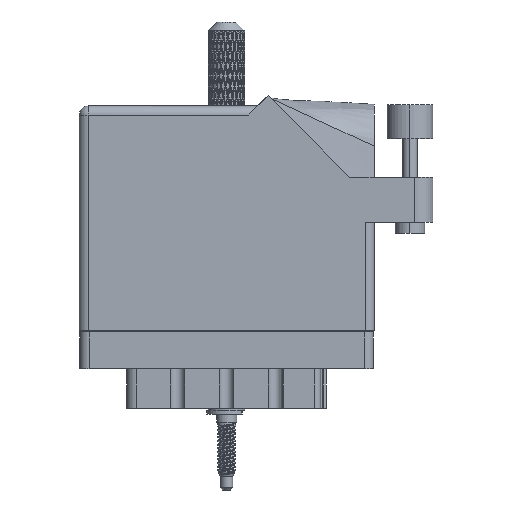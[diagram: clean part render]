
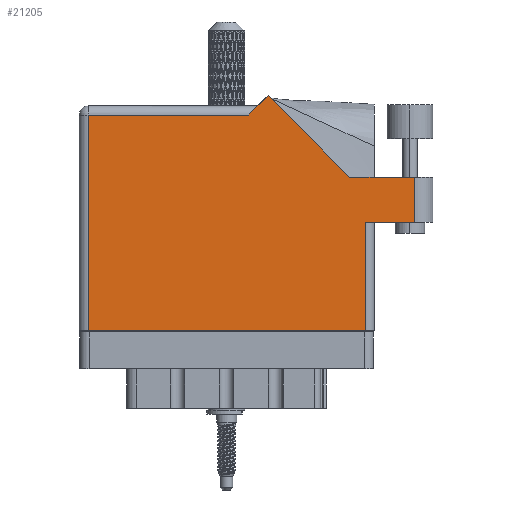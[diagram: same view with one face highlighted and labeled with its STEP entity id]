
A CAD part, front view. The second image highlights one B-rep face of the part: STEP entity #21205.
In plain terms, the highlighted face is planar.
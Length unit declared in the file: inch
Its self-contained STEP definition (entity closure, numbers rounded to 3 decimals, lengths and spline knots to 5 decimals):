
#4495 = LINE ( 'NONE', #63490, #35929 ) ;
#10375 = VERTEX_POINT ( 'NONE', #66895 ) ;
#10689 = CARTESIAN_POINT ( 'NONE',  ( 1.948, 0.737, 0. ) ) ;
#11623 = DIRECTION ( 'NONE',  ( 1., 0., 0. ) ) ;
#13002 = DIRECTION ( 'NONE',  ( 0., 1., 0. ) ) ;
#14336 = ORIENTED_EDGE ( 'NONE', *, *, #63837, .T. ) ;
#14407 = EDGE_CURVE ( 'NONE', #24327, #50296, #42086, .T. ) ;
#15687 = LINE ( 'NONE', #63874, #23790 ) ;
#17884 = CARTESIAN_POINT ( 'NONE',  ( 0.062, 1.468, 0. ) ) ;
#19351 = VERTEX_POINT ( 'NONE', #10689 ) ;
#20363 = DIRECTION ( 'NONE',  ( 0., 0., -1. ) ) ;
#20901 = DIRECTION ( 'NONE',  ( 1., 0., 0. ) ) ;
#21122 = VECTOR ( 'NONE', #20901, 39.37008 ) ;
#21205 = ADVANCED_FACE ( 'NONE', ( #87425 ), #86884, .F. ) ;
#21917 = VECTOR ( 'NONE', #93456, 39.37008 ) ;
#23449 = LINE ( 'NONE', #47319, #48902 ) ;
#23790 = VECTOR ( 'NONE', #65472, 39.37008 ) ;
#24327 = VERTEX_POINT ( 'NONE', #24471 ) ;
#24471 = CARTESIAN_POINT ( 'NONE',  ( 1.28771, 1.60071, 0. ) ) ;
#26936 = CARTESIAN_POINT ( 'NONE',  ( 1.217, 1.53, 0. ) ) ;
#27651 = ORIENTED_EDGE ( 'NONE', *, *, #27701, .T. ) ;
#27657 = ORIENTED_EDGE ( 'NONE', *, *, #100899, .T. ) ;
#27701 = EDGE_CURVE ( 'NONE', #10375, #73435, #23449, .T. ) ;
#27808 = VERTEX_POINT ( 'NONE', #57555 ) ;
#28303 = CARTESIAN_POINT ( 'NONE',  ( 2.285, 1.044, 0. ) ) ;
#29087 = ORIENTED_EDGE ( 'NONE', *, *, #60327, .T. ) ;
#30068 = CARTESIAN_POINT ( 'NONE',  ( 0., 1.53, 0. ) ) ;
#30575 = ORIENTED_EDGE ( 'NONE', *, *, #62914, .T. ) ;
#31964 = LINE ( 'NONE', #50383, #105710 ) ;
#32577 = EDGE_CURVE ( 'NONE', #100473, #19351, #36260, .T. ) ;
#32827 = VECTOR ( 'NONE', #11623, 39.37008 ) ;
#35739 = CARTESIAN_POINT ( 'NONE',  ( 1.948, 0.737, 0. ) ) ;
#35929 = VECTOR ( 'NONE', #103557, 39.37008 ) ;
#36260 = LINE ( 'NONE', #35739, #90843 ) ;
#39691 = DIRECTION ( 'NONE',  ( 0., 1., 0. ) ) ;
#41643 = DIRECTION ( 'NONE',  ( -1., 0., 0. ) ) ;
#42086 = LINE ( 'NONE', #26936, #21917 ) ;
#42162 = ORIENTED_EDGE ( 'NONE', *, *, #98832, .T. ) ;
#46256 = CARTESIAN_POINT ( 'NONE',  ( 0.062, 0., 0. ) ) ;
#46874 = DIRECTION ( 'NONE',  ( -1., 0., 0. ) ) ;
#47319 = CARTESIAN_POINT ( 'NONE',  ( 2.285, 1.044, 0. ) ) ;
#48902 = VECTOR ( 'NONE', #39691, 39.37008 ) ;
#50296 = VERTEX_POINT ( 'NONE', #88293 ) ;
#50383 = CARTESIAN_POINT ( 'NONE',  ( 1.84442, 1.044, 0. ) ) ;
#52467 = LINE ( 'NONE', #91960, #94427 ) ;
#57555 = CARTESIAN_POINT ( 'NONE',  ( 1.84442, 1.044, 0. ) ) ;
#60327 = EDGE_CURVE ( 'NONE', #50296, #80232, #4495, .T. ) ;
#62914 = EDGE_CURVE ( 'NONE', #80232, #82611, #15687, .T. ) ;
#63490 = CARTESIAN_POINT ( 'NONE',  ( 0., 1.468, 0. ) ) ;
#63837 = EDGE_CURVE ( 'NONE', #73435, #27808, #52467, .T. ) ;
#63874 = CARTESIAN_POINT ( 'NONE',  ( 0.062, 0., 0. ) ) ;
#65472 = DIRECTION ( 'NONE',  ( 0., -1., 0. ) ) ;
#66895 = CARTESIAN_POINT ( 'NONE',  ( 2.285, 0.737, 0. ) ) ;
#73435 = VERTEX_POINT ( 'NONE', #28303 ) ;
#73473 = ORIENTED_EDGE ( 'NONE', *, *, #76615, .T. ) ;
#73969 = ORIENTED_EDGE ( 'NONE', *, *, #32577, .T. ) ;
#76615 = EDGE_CURVE ( 'NONE', #19351, #10375, #86787, .T. ) ;
#80232 = VERTEX_POINT ( 'NONE', #17884 ) ;
#80323 = ORIENTED_EDGE ( 'NONE', *, *, #14407, .T. ) ;
#82611 = VERTEX_POINT ( 'NONE', #46256 ) ;
#85336 = AXIS2_PLACEMENT_3D ( 'NONE', #30068, #20363, #46874 ) ;
#85748 = CARTESIAN_POINT ( 'NONE',  ( 2.01, 0.737, 0. ) ) ;
#86787 = LINE ( 'NONE', #85748, #32827 ) ;
#86884 = PLANE ( 'NONE',  #85336 ) ;
#87425 = FACE_OUTER_BOUND ( 'NONE', #89084, .T. ) ;
#88293 = CARTESIAN_POINT ( 'NONE',  ( 1.155, 1.468, 0. ) ) ;
#89084 = EDGE_LOOP ( 'NONE', ( #73473, #27651, #14336, #42162, #80323, #29087, #30575, #27657, #73969 ) ) ;
#90843 = VECTOR ( 'NONE', #13002, 39.37008 ) ;
#91960 = CARTESIAN_POINT ( 'NONE',  ( 2.41, 1.044, 0. ) ) ;
#93456 = DIRECTION ( 'NONE',  ( -0.707, -0.707, 0. ) ) ;
#94427 = VECTOR ( 'NONE', #41643, 39.37008 ) ;
#95035 = LINE ( 'NONE', #106766, #21122 ) ;
#98832 = EDGE_CURVE ( 'NONE', #27808, #24327, #31964, .T. ) ;
#99080 = DIRECTION ( 'NONE',  ( -0.707, 0.707, 0. ) ) ;
#100473 = VERTEX_POINT ( 'NONE', #104906 ) ;
#100899 = EDGE_CURVE ( 'NONE', #82611, #100473, #95035, .T. ) ;
#103557 = DIRECTION ( 'NONE',  ( -1., 0., 0. ) ) ;
#104906 = CARTESIAN_POINT ( 'NONE',  ( 1.948, 0., 0. ) ) ;
#105710 = VECTOR ( 'NONE', #99080, 39.37008 ) ;
#106766 = CARTESIAN_POINT ( 'NONE',  ( 0., 0., 0. ) ) ;
